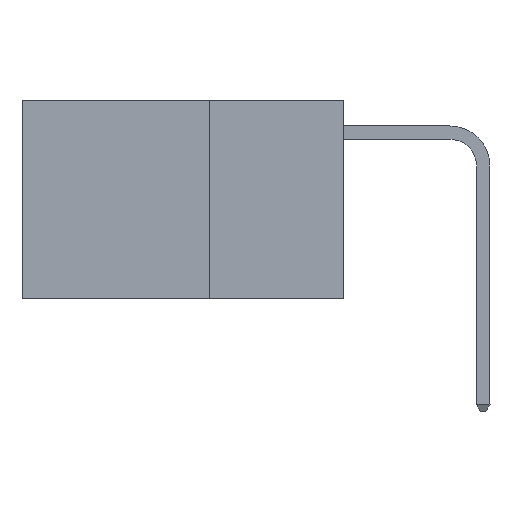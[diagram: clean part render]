
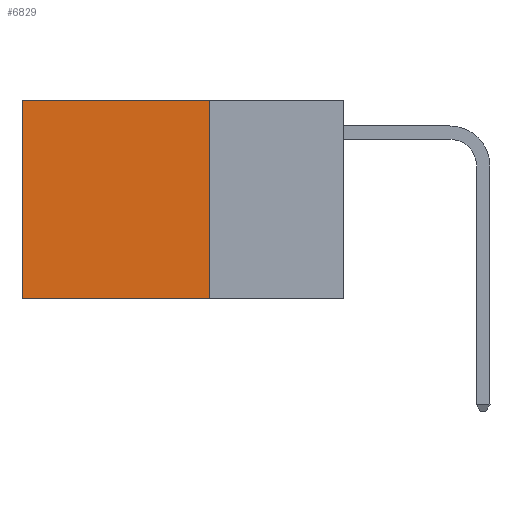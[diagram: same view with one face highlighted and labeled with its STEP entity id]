
A CAD part, left-side view. The second image highlights one B-rep face of the part: STEP entity #6829.
In plain terms, the highlighted planar face has unit normal (-1, 0, 0).
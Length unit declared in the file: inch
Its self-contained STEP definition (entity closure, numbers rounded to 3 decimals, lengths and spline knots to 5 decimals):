
#1272 = ORIENTED_EDGE ( 'NONE', *, *, #4243, .F. ) ;
#1896 = DIRECTION ( 'NONE',  ( 0., 0., -1. ) ) ;
#1996 = CARTESIAN_POINT ( 'NONE',  ( 0.2625, 0.25, 0. ) ) ;
#2008 = DIRECTION ( 'NONE',  ( 0., 1., 0. ) ) ;
#2327 = LINE ( 'NONE', #12203, #16589 ) ;
#2460 = PLANE ( 'NONE',  #16580 ) ;
#4179 = CARTESIAN_POINT ( 'NONE',  ( 0.2625, 0.6, 0. ) ) ;
#4243 = EDGE_CURVE ( 'NONE', #8801, #6259, #2327, .T. ) ;
#4489 = EDGE_CURVE ( 'NONE', #11103, #8801, #12664, .T. ) ;
#4686 = ORIENTED_EDGE ( 'NONE', *, *, #4489, .F. ) ;
#4937 = CARTESIAN_POINT ( 'NONE',  ( 0.2625, 0.25, 0. ) ) ;
#5044 = CARTESIAN_POINT ( 'NONE',  ( 0.2625, 0.25, 0. ) ) ;
#6259 = VERTEX_POINT ( 'NONE', #9650 ) ;
#6554 = FACE_OUTER_BOUND ( 'NONE', #17520, .T. ) ;
#6829 = ADVANCED_FACE ( 'NONE', ( #6554 ), #2460, .F. ) ;
#6842 = DIRECTION ( 'NONE',  ( 1., 0., 0. ) ) ;
#7007 = CARTESIAN_POINT ( 'NONE',  ( 0.2625, 0.6, 0. ) ) ;
#7249 = EDGE_CURVE ( 'NONE', #11103, #11392, #18130, .T. ) ;
#7566 = EDGE_CURVE ( 'NONE', #11392, #6259, #16231, .T. ) ;
#8801 = VERTEX_POINT ( 'NONE', #14224 ) ;
#9650 = CARTESIAN_POINT ( 'NONE',  ( 0.2625, 0.6, -0.37 ) ) ;
#11103 = VERTEX_POINT ( 'NONE', #5044 ) ;
#11392 = VERTEX_POINT ( 'NONE', #4179 ) ;
#11415 = DIRECTION ( 'NONE',  ( 0., 1., 0. ) ) ;
#12203 = CARTESIAN_POINT ( 'NONE',  ( 0.2625, 0.25, -0.37 ) ) ;
#12544 = VECTOR ( 'NONE', #14076, 39.37008 ) ;
#12664 = LINE ( 'NONE', #1996, #13545 ) ;
#13545 = VECTOR ( 'NONE', #1896, 39.37008 ) ;
#14076 = DIRECTION ( 'NONE',  ( 0., 0., -1. ) ) ;
#14224 = CARTESIAN_POINT ( 'NONE',  ( 0.2625, 0.25, -0.37 ) ) ;
#14498 = VECTOR ( 'NONE', #2008, 39.37008 ) ;
#15328 = CARTESIAN_POINT ( 'NONE',  ( 0.2625, 0.25, 0. ) ) ;
#16175 = ORIENTED_EDGE ( 'NONE', *, *, #7249, .T. ) ;
#16231 = LINE ( 'NONE', #7007, #12544 ) ;
#16580 = AXIS2_PLACEMENT_3D ( 'NONE', #15328, #6842, #16726 ) ;
#16589 = VECTOR ( 'NONE', #11415, 39.37008 ) ;
#16726 = DIRECTION ( 'NONE',  ( 0., 0., -1. ) ) ;
#17520 = EDGE_LOOP ( 'NONE', ( #17782, #1272, #4686, #16175 ) ) ;
#17782 = ORIENTED_EDGE ( 'NONE', *, *, #7566, .T. ) ;
#18130 = LINE ( 'NONE', #4937, #14498 ) ;
